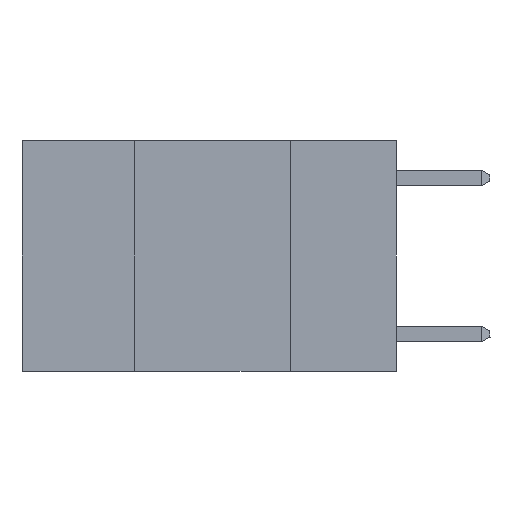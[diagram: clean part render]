
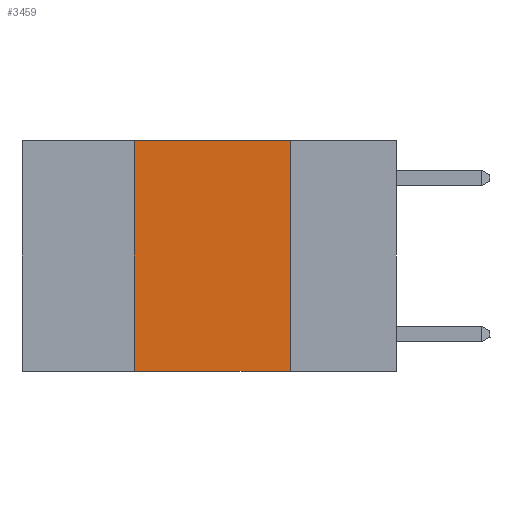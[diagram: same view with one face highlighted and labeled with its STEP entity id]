
A CAD part, left-side view. The second image highlights one B-rep face of the part: STEP entity #3459.
In plain terms, the highlighted planar face has unit normal (-1, 0, 0).
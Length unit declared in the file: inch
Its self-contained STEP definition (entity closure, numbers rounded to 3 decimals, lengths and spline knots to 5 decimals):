
#40 = LINE ( 'NONE', #14249, #11845 ) ;
#1505 = VERTEX_POINT ( 'NONE', #6342 ) ;
#1581 = DIRECTION ( 'NONE',  ( 0., 0., -1. ) ) ;
#1805 = EDGE_CURVE ( 'NONE', #1505, #5000, #8469, .T. ) ;
#2535 = AXIS2_PLACEMENT_3D ( 'NONE', #14345, #13275, #6792 ) ;
#3230 = DIRECTION ( 'NONE',  ( 0., -1., 0. ) ) ;
#3423 = EDGE_CURVE ( 'NONE', #11345, #13858, #40, .T. ) ;
#3459 = ADVANCED_FACE ( 'NONE', ( #11524 ), #4362, .F. ) ;
#4362 = PLANE ( 'NONE',  #2535 ) ;
#4518 = LINE ( 'NONE', #11971, #12402 ) ;
#5000 = VERTEX_POINT ( 'NONE', #11374 ) ;
#5449 = VECTOR ( 'NONE', #1581, 39.37008 ) ;
#6342 = CARTESIAN_POINT ( 'NONE',  ( 0., 0.42, 0. ) ) ;
#6792 = DIRECTION ( 'NONE',  ( 0., 0., -1. ) ) ;
#6877 = CARTESIAN_POINT ( 'NONE',  ( 0., 0.6, 0. ) ) ;
#7328 = EDGE_CURVE ( 'NONE', #11345, #1505, #4518, .T. ) ;
#7496 = CARTESIAN_POINT ( 'NONE',  ( 0., 0.17, 0. ) ) ;
#7904 = ORIENTED_EDGE ( 'NONE', *, *, #7328, .F. ) ;
#8110 = ORIENTED_EDGE ( 'NONE', *, *, #3423, .T. ) ;
#8469 = LINE ( 'NONE', #6877, #13884 ) ;
#8678 = ORIENTED_EDGE ( 'NONE', *, *, #1805, .F. ) ;
#8763 = DIRECTION ( 'NONE',  ( 0., 0., 1. ) ) ;
#9016 = ORIENTED_EDGE ( 'NONE', *, *, #11523, .F. ) ;
#9477 = CARTESIAN_POINT ( 'NONE',  ( 0., 0.42, -0.37 ) ) ;
#9958 = DIRECTION ( 'NONE',  ( 0., -1., 0. ) ) ;
#11345 = VERTEX_POINT ( 'NONE', #9477 ) ;
#11374 = CARTESIAN_POINT ( 'NONE',  ( 0., 0.17, 0. ) ) ;
#11380 = EDGE_LOOP ( 'NONE', ( #9016, #8678, #7904, #8110 ) ) ;
#11389 = LINE ( 'NONE', #7496, #5449 ) ;
#11523 = EDGE_CURVE ( 'NONE', #5000, #13858, #11389, .T. ) ;
#11524 = FACE_OUTER_BOUND ( 'NONE', #11380, .T. ) ;
#11845 = VECTOR ( 'NONE', #9958, 39.37008 ) ;
#11971 = CARTESIAN_POINT ( 'NONE',  ( 0., 0.42, 0. ) ) ;
#12402 = VECTOR ( 'NONE', #8763, 39.37008 ) ;
#13275 = DIRECTION ( 'NONE',  ( 1., 0., 0. ) ) ;
#13858 = VERTEX_POINT ( 'NONE', #14289 ) ;
#13884 = VECTOR ( 'NONE', #3230, 39.37008 ) ;
#14249 = CARTESIAN_POINT ( 'NONE',  ( 0., 0.6, -0.37 ) ) ;
#14289 = CARTESIAN_POINT ( 'NONE',  ( 0., 0.17, -0.37 ) ) ;
#14345 = CARTESIAN_POINT ( 'NONE',  ( 0., 0.6, 0. ) ) ;
